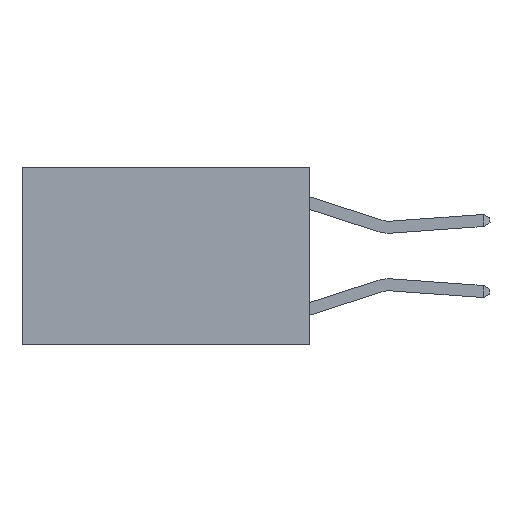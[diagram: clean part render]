
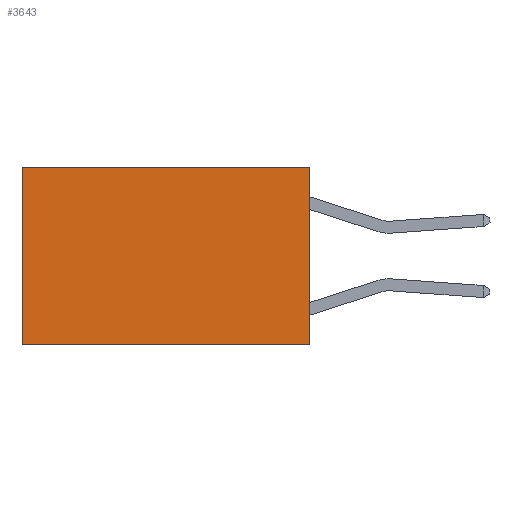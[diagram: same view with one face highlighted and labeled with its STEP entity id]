
A CAD part, left-side view. The second image highlights one B-rep face of the part: STEP entity #3643.
In plain terms, the highlighted planar face has unit normal (-1, 0, 0).
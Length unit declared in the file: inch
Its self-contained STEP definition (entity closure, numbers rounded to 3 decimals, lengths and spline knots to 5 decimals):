
#1103 = CARTESIAN_POINT ( 'NONE',  ( 0.2625, 0., -0.37 ) ) ;
#1610 = ORIENTED_EDGE ( 'NONE', *, *, #12711, .T. ) ;
#1820 = LINE ( 'NONE', #10434, #5314 ) ;
#1882 = DIRECTION ( 'NONE',  ( 0., 0., -1. ) ) ;
#2293 = AXIS2_PLACEMENT_3D ( 'NONE', #14679, #16149, #7394 ) ;
#3079 = LINE ( 'NONE', #12197, #13840 ) ;
#3177 = VERTEX_POINT ( 'NONE', #12114 ) ;
#3426 = DIRECTION ( 'NONE',  ( 0., 0., -1. ) ) ;
#3460 = CARTESIAN_POINT ( 'NONE',  ( 0.2625, 0., -0.37 ) ) ;
#3643 = ADVANCED_FACE ( 'NONE', ( #13173 ), #4435, .F. ) ;
#4435 = PLANE ( 'NONE',  #2293 ) ;
#4741 = VECTOR ( 'NONE', #3426, 39.37008 ) ;
#4784 = VERTEX_POINT ( 'NONE', #1103 ) ;
#5192 = EDGE_CURVE ( 'NONE', #11379, #4784, #11647, .T. ) ;
#5314 = VECTOR ( 'NONE', #16226, 39.37008 ) ;
#6014 = VERTEX_POINT ( 'NONE', #8348 ) ;
#6016 = ORIENTED_EDGE ( 'NONE', *, *, #6428, .T. ) ;
#6191 = VECTOR ( 'NONE', #13192, 39.37008 ) ;
#6192 = ORIENTED_EDGE ( 'NONE', *, *, #13995, .F. ) ;
#6428 = EDGE_CURVE ( 'NONE', #3177, #6014, #3079, .T. ) ;
#6512 = EDGE_LOOP ( 'NONE', ( #6016, #6192, #14505, #1610 ) ) ;
#7394 = DIRECTION ( 'NONE',  ( 0., 0., -1. ) ) ;
#8348 = CARTESIAN_POINT ( 'NONE',  ( 0.2625, 0.6, -0.37 ) ) ;
#8721 = CARTESIAN_POINT ( 'NONE',  ( 0.2625, 0., 0. ) ) ;
#10434 = CARTESIAN_POINT ( 'NONE',  ( 0.2625, 0., 0. ) ) ;
#11379 = VERTEX_POINT ( 'NONE', #8721 ) ;
#11647 = LINE ( 'NONE', #18029, #4741 ) ;
#12114 = CARTESIAN_POINT ( 'NONE',  ( 0.2625, 0.6, 0. ) ) ;
#12197 = CARTESIAN_POINT ( 'NONE',  ( 0.2625, 0.6, 0. ) ) ;
#12711 = EDGE_CURVE ( 'NONE', #11379, #3177, #1820, .T. ) ;
#13173 = FACE_OUTER_BOUND ( 'NONE', #6512, .T. ) ;
#13192 = DIRECTION ( 'NONE',  ( 0., 1., 0. ) ) ;
#13488 = LINE ( 'NONE', #3460, #6191 ) ;
#13840 = VECTOR ( 'NONE', #1882, 39.37008 ) ;
#13995 = EDGE_CURVE ( 'NONE', #4784, #6014, #13488, .T. ) ;
#14505 = ORIENTED_EDGE ( 'NONE', *, *, #5192, .F. ) ;
#14679 = CARTESIAN_POINT ( 'NONE',  ( 0.2625, 0., 0. ) ) ;
#16149 = DIRECTION ( 'NONE',  ( 1., 0., 0. ) ) ;
#16226 = DIRECTION ( 'NONE',  ( 0., 1., 0. ) ) ;
#18029 = CARTESIAN_POINT ( 'NONE',  ( 0.2625, 0., 0. ) ) ;
